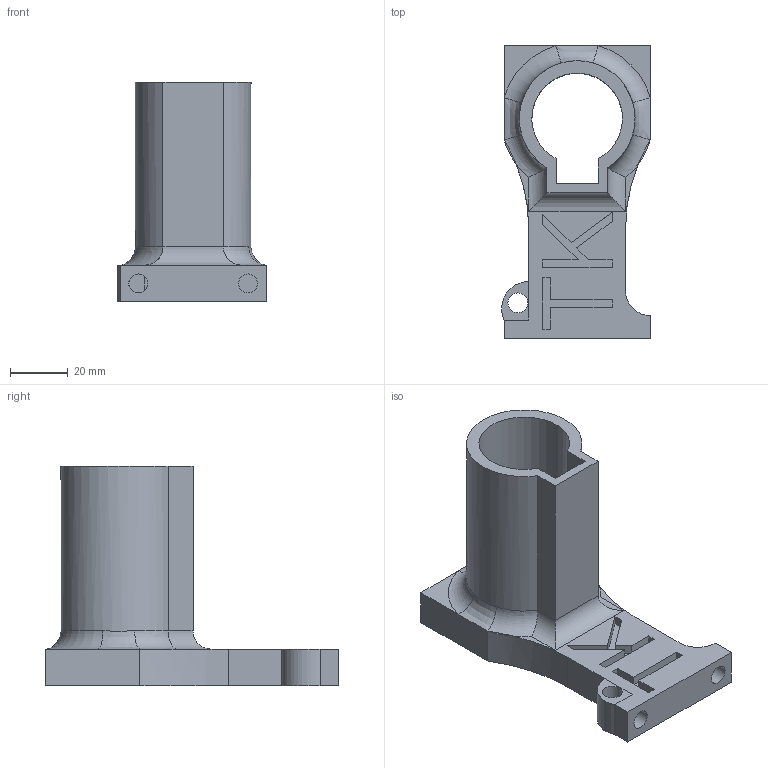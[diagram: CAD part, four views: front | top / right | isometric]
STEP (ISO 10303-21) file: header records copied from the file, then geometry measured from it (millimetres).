
FILE_DESCRIPTION(('FreeCAD Model'),'2;1');
FILE_NAME( 'DAVID-pull.step', '2018-08-24T11:18:14',('Author'),(''), 'Open CASCADE STEP processor 6.8','FreeCAD','Unknown');
FILE_SCHEMA(('AUTOMOTIVE_DESIGN_CC2 { 1 2 10303 214 -1 1 5 4 }'));
Length unit declared in the file: millimetre
Products named in the file (1): Pad002
Bounding box: 51.61 x 101.6 x 76.2 mm (x, y, z)
Volume: 75475.2 mm3; surface area: 31484.7 mm2
Topology: 1 solids, 1 shells, 384 faces, 1036 edges, 686 vertices
Faces by surface type: plane 214, extrusion 148, cylinder 15, torus 4, bspline 3
Full cylindrical faces by diameter (mm): 6.604 x4, 6.858 x1
Entity records: 26448 total; most frequent: CARTESIAN_POINT 6670, DIRECTION 3108, VECTOR 2536, LINE 2388, ORIENTED_EDGE 2072, PCURVE 2072, DEFINITIONAL_REPRESENTATION 2072, EDGE_CURVE 1036
